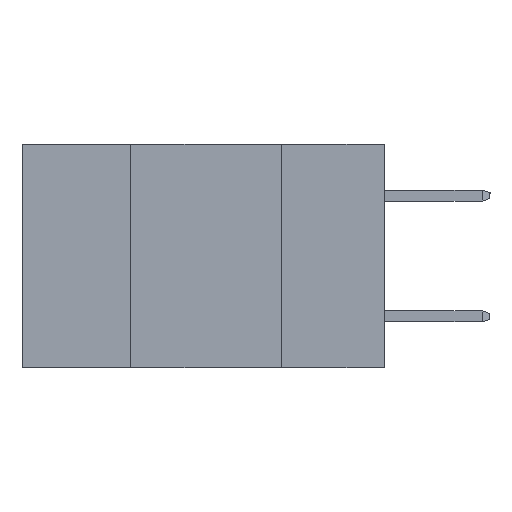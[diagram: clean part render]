
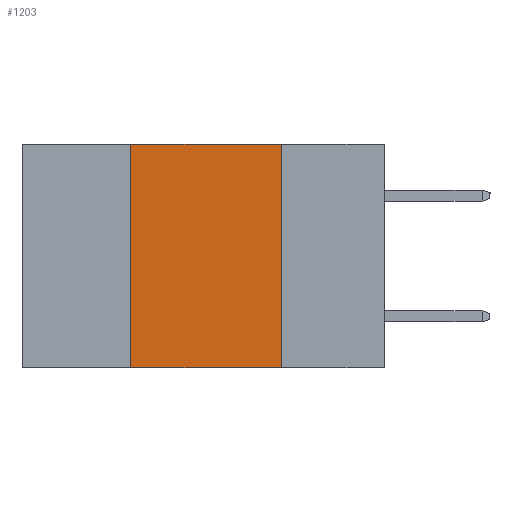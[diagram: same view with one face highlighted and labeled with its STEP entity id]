
A CAD part, left-side view. The second image highlights one B-rep face of the part: STEP entity #1203.
In plain terms, the highlighted planar face has unit normal (-1, 0, 0).
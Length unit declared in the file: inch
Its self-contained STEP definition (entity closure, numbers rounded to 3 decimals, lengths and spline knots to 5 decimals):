
#552 = CARTESIAN_POINT ( 'NONE',  ( 0., 0.6, -0.37 ) ) ;
#790 = VECTOR ( 'NONE', #3727, 39.37008 ) ;
#917 = VECTOR ( 'NONE', #4112, 39.37008 ) ;
#926 = LINE ( 'NONE', #975, #1395 ) ;
#975 = CARTESIAN_POINT ( 'NONE',  ( 0., 0.6, 0. ) ) ;
#1120 = DIRECTION ( 'NONE',  ( 0., -1., 0. ) ) ;
#1203 = ADVANCED_FACE ( 'NONE', ( #4204 ), #3312, .F. ) ;
#1395 = VECTOR ( 'NONE', #1120, 39.37008 ) ;
#1406 = AXIS2_PLACEMENT_3D ( 'NONE', #7049, #6862, #6172 ) ;
#1468 = CARTESIAN_POINT ( 'NONE',  ( 0., 0.42, 0. ) ) ;
#1813 = LINE ( 'NONE', #552, #5579 ) ;
#1831 = VERTEX_POINT ( 'NONE', #3902 ) ;
#2395 = CARTESIAN_POINT ( 'NONE',  ( 0., 0.17, 0. ) ) ;
#2616 = DIRECTION ( 'NONE',  ( 0., -1., 0. ) ) ;
#3097 = CARTESIAN_POINT ( 'NONE',  ( 0., 0.42, -0.37 ) ) ;
#3312 = PLANE ( 'NONE',  #1406 ) ;
#3540 = LINE ( 'NONE', #6252, #917 ) ;
#3727 = DIRECTION ( 'NONE',  ( 0., 0., 1. ) ) ;
#3902 = CARTESIAN_POINT ( 'NONE',  ( 0., 0.17, -0.37 ) ) ;
#4112 = DIRECTION ( 'NONE',  ( 0., 0., -1. ) ) ;
#4204 = FACE_OUTER_BOUND ( 'NONE', #7667, .T. ) ;
#4216 = ORIENTED_EDGE ( 'NONE', *, *, #4790, .F. ) ;
#4459 = EDGE_CURVE ( 'NONE', #6310, #1831, #1813, .T. ) ;
#4790 = EDGE_CURVE ( 'NONE', #5219, #1831, #3540, .T. ) ;
#5219 = VERTEX_POINT ( 'NONE', #2395 ) ;
#5579 = VECTOR ( 'NONE', #2616, 39.37008 ) ;
#6172 = DIRECTION ( 'NONE',  ( 0., 0., -1. ) ) ;
#6252 = CARTESIAN_POINT ( 'NONE',  ( 0., 0.17, -0.37 ) ) ;
#6310 = VERTEX_POINT ( 'NONE', #6916 ) ;
#6371 = VERTEX_POINT ( 'NONE', #1468 ) ;
#6576 = EDGE_CURVE ( 'NONE', #6310, #6371, #8092, .T. ) ;
#6862 = DIRECTION ( 'NONE',  ( 1., 0., 0. ) ) ;
#6916 = CARTESIAN_POINT ( 'NONE',  ( 0., 0.42, -0.37 ) ) ;
#6925 = EDGE_CURVE ( 'NONE', #6371, #5219, #926, .T. ) ;
#7049 = CARTESIAN_POINT ( 'NONE',  ( 0., 0.6, 0. ) ) ;
#7667 = EDGE_LOOP ( 'NONE', ( #4216, #8872, #8865, #8307 ) ) ;
#8092 = LINE ( 'NONE', #3097, #790 ) ;
#8307 = ORIENTED_EDGE ( 'NONE', *, *, #4459, .T. ) ;
#8865 = ORIENTED_EDGE ( 'NONE', *, *, #6576, .F. ) ;
#8872 = ORIENTED_EDGE ( 'NONE', *, *, #6925, .F. ) ;
